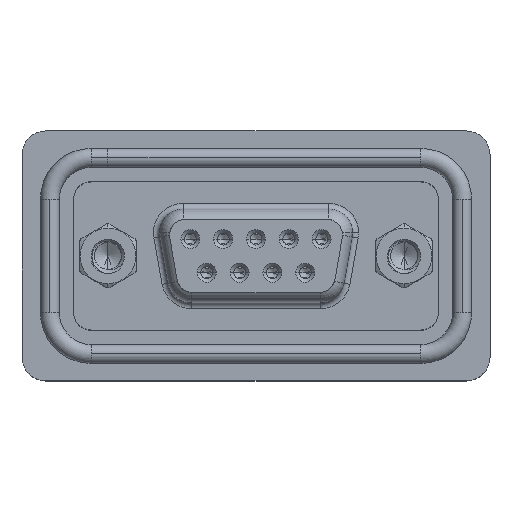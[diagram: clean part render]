
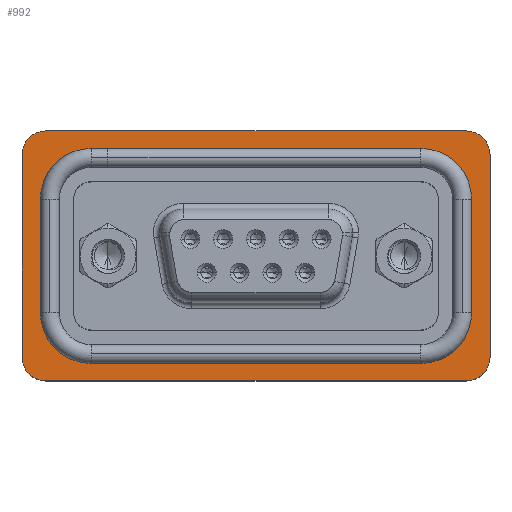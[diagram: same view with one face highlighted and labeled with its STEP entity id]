
A CAD part, top view. The second image highlights one B-rep face of the part: STEP entity #992.
In plain terms, the highlighted planar face has unit normal (0, 0, 1).
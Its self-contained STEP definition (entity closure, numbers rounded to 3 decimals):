
#41 = CARTESIAN_POINT ( 'NONE',  ( -5.25, 8.55, 0.5 ) ) ;
#280 = CIRCLE ( 'NONE', #12154, 4.3 ) ;
#281 = VECTOR ( 'NONE', #5358, 1000. ) ;
#459 = CIRCLE ( 'NONE', #12673, 2. ) ;
#537 = VERTEX_POINT ( 'NONE', #19742 ) ;
#618 = LINE ( 'NONE', #8942, #14205 ) ;
#682 = VERTEX_POINT ( 'NONE', #20577 ) ;
#740 = CARTESIAN_POINT ( 'NONE',  ( 32.25, -8.55, 0.5 ) ) ;
#825 = EDGE_LOOP ( 'NONE', ( #15680, #15686, #11358, #15724, #4077, #6945, #21493, #18635 ) ) ;
#992 = ADVANCED_FACE ( 'NONE', ( #9884, #5189 ), #11842, .T. ) ;
#1010 = DIRECTION ( 'NONE',  ( 0., 0., 1. ) ) ;
#1015 = CARTESIAN_POINT ( 'NONE',  ( -7.25, -8.55, 0.5 ) ) ;
#1555 = DIRECTION ( 'NONE',  ( 0., 0., 1. ) ) ;
#1753 = EDGE_CURVE ( 'NONE', #682, #7825, #280, .T. ) ;
#1779 = VERTEX_POINT ( 'NONE', #16250 ) ;
#1959 = CARTESIAN_POINT ( 'NONE',  ( 32.25, -8.55, 0.5 ) ) ;
#1977 = EDGE_CURVE ( 'NONE', #7825, #17729, #5354, .T. ) ;
#2034 = VERTEX_POINT ( 'NONE', #740 ) ;
#2061 = DIRECTION ( 'NONE',  ( 0., 0., 1. ) ) ;
#2284 = DIRECTION ( 'NONE',  ( 0., 1., 0. ) ) ;
#2546 = VECTOR ( 'NONE', #17418, 1000. ) ;
#3224 = CIRCLE ( 'NONE', #20661, 4.3 ) ;
#3608 = CARTESIAN_POINT ( 'NONE',  ( 30.25, -8.55, 0.5 ) ) ;
#3649 = VERTEX_POINT ( 'NONE', #21128 ) ;
#3657 = DIRECTION ( 'NONE',  ( -1., 0., 0. ) ) ;
#3754 = AXIS2_PLACEMENT_3D ( 'NONE', #10212, #1555, #15208 ) ;
#3904 = CARTESIAN_POINT ( 'NONE',  ( 30.7, -4.775, 0.5 ) ) ;
#4049 = LINE ( 'NONE', #20730, #16737 ) ;
#4077 = ORIENTED_EDGE ( 'NONE', *, *, #1753, .F. ) ;
#5050 = VERTEX_POINT ( 'NONE', #15321 ) ;
#5095 = DIRECTION ( 'NONE',  ( 1., 0., 0. ) ) ;
#5189 = FACE_OUTER_BOUND ( 'NONE', #17673, .T. ) ;
#5354 = LINE ( 'NONE', #18636, #15612 ) ;
#5358 = DIRECTION ( 'NONE',  ( 0., 1., 0. ) ) ;
#5667 = CARTESIAN_POINT ( 'NONE',  ( -1.4, -9.075, 0.5 ) ) ;
#6128 = CARTESIAN_POINT ( 'NONE',  ( 26.4, 4.775, 0.5 ) ) ;
#6486 = VERTEX_POINT ( 'NONE', #18905 ) ;
#6607 = AXIS2_PLACEMENT_3D ( 'NONE', #21169, #16239, #14833 ) ;
#6886 = EDGE_CURVE ( 'NONE', #18931, #3649, #17140, .T. ) ;
#6945 = ORIENTED_EDGE ( 'NONE', *, *, #15075, .F. ) ;
#7205 = CARTESIAN_POINT ( 'NONE',  ( 26.4, -9.075, 0.5 ) ) ;
#7216 = CIRCLE ( 'NONE', #7920, 2. ) ;
#7296 = CARTESIAN_POINT ( 'NONE',  ( 30.25, -10.55, 0.5 ) ) ;
#7510 = VECTOR ( 'NONE', #8890, 1000. ) ;
#7529 = CARTESIAN_POINT ( 'NONE',  ( 30.25, 10.55, 0.5 ) ) ;
#7559 = VERTEX_POINT ( 'NONE', #17556 ) ;
#7785 = CARTESIAN_POINT ( 'NONE',  ( 30.25, -10.55, 0.5 ) ) ;
#7825 = VERTEX_POINT ( 'NONE', #5667 ) ;
#7854 = VERTEX_POINT ( 'NONE', #3904 ) ;
#7920 = AXIS2_PLACEMENT_3D ( 'NONE', #13817, #18579, #3657 ) ;
#8098 = AXIS2_PLACEMENT_3D ( 'NONE', #3608, #2061, #8424 ) ;
#8372 = VECTOR ( 'NONE', #19341, 1000. ) ;
#8424 = DIRECTION ( 'NONE',  ( 1., 0., 0. ) ) ;
#8678 = CARTESIAN_POINT ( 'NONE',  ( -1.4, 4.775, 0.5 ) ) ;
#8724 = ORIENTED_EDGE ( 'NONE', *, *, #20958, .T. ) ;
#8890 = DIRECTION ( 'NONE',  ( -1., 0., 0. ) ) ;
#8942 = CARTESIAN_POINT ( 'NONE',  ( 26.4, 9.075, 0.5 ) ) ;
#9050 = LINE ( 'NONE', #12421, #2546 ) ;
#9053 = CIRCLE ( 'NONE', #6607, 4.3 ) ;
#9744 = ORIENTED_EDGE ( 'NONE', *, *, #10192, .T. ) ;
#9756 = LINE ( 'NONE', #1015, #8372 ) ;
#9884 = FACE_BOUND ( 'NONE', #825, .T. ) ;
#9916 = CIRCLE ( 'NONE', #17893, 4.3 ) ;
#10192 = EDGE_CURVE ( 'NONE', #7559, #537, #7216, .T. ) ;
#10212 = CARTESIAN_POINT ( 'NONE',  ( 30.25, 8.55, 0.5 ) ) ;
#10567 = AXIS2_PLACEMENT_3D ( 'NONE', #19331, #1010, #17142 ) ;
#10677 = DIRECTION ( 'NONE',  ( -1., 0., 0. ) ) ;
#11045 = CARTESIAN_POINT ( 'NONE',  ( -1.4, -4.775, 0.5 ) ) ;
#11098 = EDGE_CURVE ( 'NONE', #16383, #5050, #618, .T. ) ;
#11358 = ORIENTED_EDGE ( 'NONE', *, *, #20093, .F. ) ;
#11842 = PLANE ( 'NONE',  #3754 ) ;
#11967 = DIRECTION ( 'NONE',  ( 0., 0., 1. ) ) ;
#12113 = DIRECTION ( 'NONE',  ( 1., 0., 0. ) ) ;
#12154 = AXIS2_PLACEMENT_3D ( 'NONE', #11045, #14535, #16145 ) ;
#12297 = VERTEX_POINT ( 'NONE', #7785 ) ;
#12305 = CARTESIAN_POINT ( 'NONE',  ( 26.4, 9.075, 0.5 ) ) ;
#12401 = EDGE_CURVE ( 'NONE', #2034, #6486, #19638, .T. ) ;
#12421 = CARTESIAN_POINT ( 'NONE',  ( -5.7, 4.775, 0.5 ) ) ;
#12673 = AXIS2_PLACEMENT_3D ( 'NONE', #41, #11967, #5095 ) ;
#12777 = DIRECTION ( 'NONE',  ( 0., 0., 1. ) ) ;
#12969 = ORIENTED_EDGE ( 'NONE', *, *, #16883, .T. ) ;
#12980 = VECTOR ( 'NONE', #20369, 1000. ) ;
#13590 = EDGE_CURVE ( 'NONE', #12297, #2034, #14013, .T. ) ;
#13817 = CARTESIAN_POINT ( 'NONE',  ( -5.25, -8.55, 0.5 ) ) ;
#14013 = CIRCLE ( 'NONE', #8098, 2. ) ;
#14135 = EDGE_CURVE ( 'NONE', #537, #12297, #17197, .T. ) ;
#14205 = VECTOR ( 'NONE', #10677, 1000. ) ;
#14535 = DIRECTION ( 'NONE',  ( 0., 0., 1. ) ) ;
#14833 = DIRECTION ( 'NONE',  ( 1., 0., 0. ) ) ;
#15075 = EDGE_CURVE ( 'NONE', #15211, #682, #9050, .T. ) ;
#15208 = DIRECTION ( 'NONE',  ( 1., 0., 0. ) ) ;
#15211 = VERTEX_POINT ( 'NONE', #21025 ) ;
#15304 = DIRECTION ( 'NONE',  ( 0., 0., 1. ) ) ;
#15321 = CARTESIAN_POINT ( 'NONE',  ( -1.4, 9.075, 0.5 ) ) ;
#15493 = EDGE_CURVE ( 'NONE', #3649, #21115, #459, .T. ) ;
#15612 = VECTOR ( 'NONE', #12113, 1000. ) ;
#15680 = ORIENTED_EDGE ( 'NONE', *, *, #16034, .F. ) ;
#15686 = ORIENTED_EDGE ( 'NONE', *, *, #19499, .F. ) ;
#15724 = ORIENTED_EDGE ( 'NONE', *, *, #1977, .F. ) ;
#15780 = CIRCLE ( 'NONE', #10567, 2. ) ;
#16034 = EDGE_CURVE ( 'NONE', #1779, #16383, #9916, .T. ) ;
#16145 = DIRECTION ( 'NONE',  ( 1., 0., 0. ) ) ;
#16239 = DIRECTION ( 'NONE',  ( 0., 0., 1. ) ) ;
#16250 = CARTESIAN_POINT ( 'NONE',  ( 30.7, 4.775, 0.5 ) ) ;
#16383 = VERTEX_POINT ( 'NONE', #12305 ) ;
#16632 = EDGE_CURVE ( 'NONE', #5050, #15211, #3224, .T. ) ;
#16737 = VECTOR ( 'NONE', #2284, 1000. ) ;
#16829 = ORIENTED_EDGE ( 'NONE', *, *, #12401, .T. ) ;
#16883 = EDGE_CURVE ( 'NONE', #6486, #18931, #15780, .T. ) ;
#17040 = CARTESIAN_POINT ( 'NONE',  ( 30.25, 10.55, 0.5 ) ) ;
#17140 = LINE ( 'NONE', #17040, #7510 ) ;
#17142 = DIRECTION ( 'NONE',  ( 1., 0., 0. ) ) ;
#17197 = LINE ( 'NONE', #7296, #12980 ) ;
#17418 = DIRECTION ( 'NONE',  ( 0., -1., 0. ) ) ;
#17556 = CARTESIAN_POINT ( 'NONE',  ( -7.25, -8.55, 0.5 ) ) ;
#17673 = EDGE_LOOP ( 'NONE', ( #12969, #20479, #19587, #8724, #9744, #20760, #21079, #16829 ) ) ;
#17729 = VERTEX_POINT ( 'NONE', #7205 ) ;
#17893 = AXIS2_PLACEMENT_3D ( 'NONE', #6128, #12777, #19297 ) ;
#18579 = DIRECTION ( 'NONE',  ( 0., 0., 1. ) ) ;
#18635 = ORIENTED_EDGE ( 'NONE', *, *, #11098, .F. ) ;
#18636 = CARTESIAN_POINT ( 'NONE',  ( -1.4, -9.075, 0.5 ) ) ;
#18905 = CARTESIAN_POINT ( 'NONE',  ( 32.25, 8.55, 0.5 ) ) ;
#18931 = VERTEX_POINT ( 'NONE', #7529 ) ;
#19297 = DIRECTION ( 'NONE',  ( 1., 0., 0. ) ) ;
#19331 = CARTESIAN_POINT ( 'NONE',  ( 30.25, 8.55, 0.5 ) ) ;
#19341 = DIRECTION ( 'NONE',  ( 0., -1., 0. ) ) ;
#19499 = EDGE_CURVE ( 'NONE', #7854, #1779, #4049, .T. ) ;
#19587 = ORIENTED_EDGE ( 'NONE', *, *, #15493, .T. ) ;
#19638 = LINE ( 'NONE', #1959, #281 ) ;
#19742 = CARTESIAN_POINT ( 'NONE',  ( -5.25, -10.55, 0.5 ) ) ;
#20093 = EDGE_CURVE ( 'NONE', #17729, #7854, #9053, .T. ) ;
#20208 = DIRECTION ( 'NONE',  ( 1., 0., 0. ) ) ;
#20369 = DIRECTION ( 'NONE',  ( 1., 0., 0. ) ) ;
#20479 = ORIENTED_EDGE ( 'NONE', *, *, #6886, .T. ) ;
#20577 = CARTESIAN_POINT ( 'NONE',  ( -5.7, -4.775, 0.5 ) ) ;
#20661 = AXIS2_PLACEMENT_3D ( 'NONE', #8678, #15304, #20208 ) ;
#20730 = CARTESIAN_POINT ( 'NONE',  ( 30.7, -4.775, 0.5 ) ) ;
#20760 = ORIENTED_EDGE ( 'NONE', *, *, #14135, .T. ) ;
#20958 = EDGE_CURVE ( 'NONE', #21115, #7559, #9756, .T. ) ;
#21025 = CARTESIAN_POINT ( 'NONE',  ( -5.7, 4.775, 0.5 ) ) ;
#21079 = ORIENTED_EDGE ( 'NONE', *, *, #13590, .T. ) ;
#21115 = VERTEX_POINT ( 'NONE', #21522 ) ;
#21128 = CARTESIAN_POINT ( 'NONE',  ( -5.25, 10.55, 0.5 ) ) ;
#21169 = CARTESIAN_POINT ( 'NONE',  ( 26.4, -4.775, 0.5 ) ) ;
#21493 = ORIENTED_EDGE ( 'NONE', *, *, #16632, .F. ) ;
#21522 = CARTESIAN_POINT ( 'NONE',  ( -7.25, 8.55, 0.5 ) ) ;
